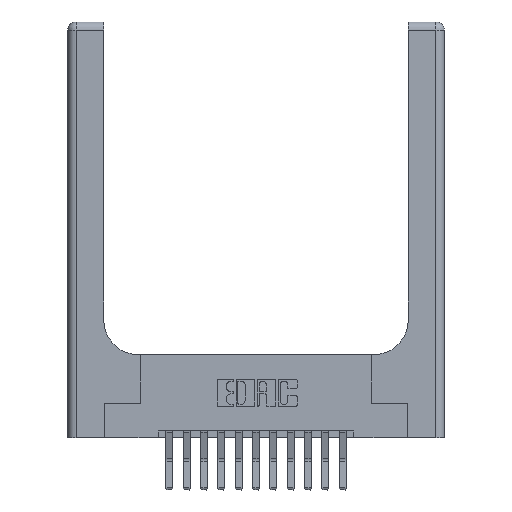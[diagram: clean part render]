
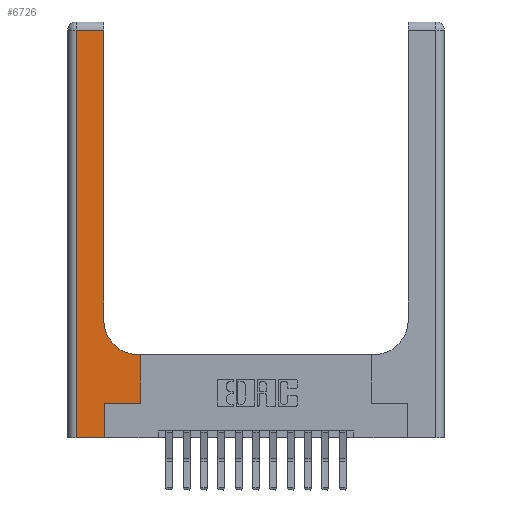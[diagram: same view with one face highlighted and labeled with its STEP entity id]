
A CAD part, top view. The second image highlights one B-rep face of the part: STEP entity #6726.
In plain terms, the highlighted planar face has unit normal (0, 0, 1).
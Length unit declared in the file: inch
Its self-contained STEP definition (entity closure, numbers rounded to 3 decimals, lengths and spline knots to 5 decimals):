
#40 = VECTOR ( 'NONE', #6164, 39.37008 ) ;
#179 = VECTOR ( 'NONE', #2635, 39.37008 ) ;
#310 = LINE ( 'NONE', #14817, #179 ) ;
#576 = ORIENTED_EDGE ( 'NONE', *, *, #7065, .T. ) ;
#774 = VECTOR ( 'NONE', #9963, 39.37008 ) ;
#799 = ORIENTED_EDGE ( 'NONE', *, *, #4863, .T. ) ;
#861 = VECTOR ( 'NONE', #8467, 39.37008 ) ;
#1094 = DIRECTION ( 'NONE',  ( 1., 0., 0. ) ) ;
#1190 = DIRECTION ( 'NONE',  ( 1., 0., 0. ) ) ;
#1558 = EDGE_CURVE ( 'NONE', #4758, #15224, #4155, .T. ) ;
#1905 = DIRECTION ( 'NONE',  ( 0., 0., -1. ) ) ;
#1984 = CARTESIAN_POINT ( 'NONE',  ( 0.265, 0., 0.37 ) ) ;
#2122 = ORIENTED_EDGE ( 'NONE', *, *, #2611, .T. ) ;
#2321 = LINE ( 'NONE', #9156, #13183 ) ;
#2480 = VERTEX_POINT ( 'NONE', #4492 ) ;
#2515 = EDGE_CURVE ( 'NONE', #2480, #12943, #10779, .T. ) ;
#2611 = EDGE_CURVE ( 'NONE', #15224, #6782, #4359, .T. ) ;
#2635 = DIRECTION ( 'NONE',  ( 0., 1., 0. ) ) ;
#2997 = LINE ( 'NONE', #5791, #774 ) ;
#3455 = CARTESIAN_POINT ( 'NONE',  ( 0.51, 0.85, 0.37 ) ) ;
#3461 = CARTESIAN_POINT ( 'NONE',  ( 0., 3., 0.37 ) ) ;
#3521 = CARTESIAN_POINT ( 'NONE',  ( 0.265, 0.25, 0.37 ) ) ;
#3657 = CARTESIAN_POINT ( 'NONE',  ( 0.528, 0.25, 0.37 ) ) ;
#4143 = EDGE_CURVE ( 'NONE', #16834, #12425, #2321, .T. ) ;
#4155 = LINE ( 'NONE', #9263, #8194 ) ;
#4359 = LINE ( 'NONE', #9868, #4423 ) ;
#4423 = VECTOR ( 'NONE', #8439, 39.37008 ) ;
#4476 = CARTESIAN_POINT ( 'NONE',  ( 0.265, 0., 0.37 ) ) ;
#4492 = CARTESIAN_POINT ( 'NONE',  ( 0.51, 0.6, 0.37 ) ) ;
#4731 = CARTESIAN_POINT ( 'NONE',  ( 0.06, 2.94, 0.37 ) ) ;
#4758 = VERTEX_POINT ( 'NONE', #4731 ) ;
#4863 = EDGE_CURVE ( 'NONE', #12943, #10801, #310, .T. ) ;
#5688 = CARTESIAN_POINT ( 'NONE',  ( 0.26, 0.85, 0.37 ) ) ;
#5791 = CARTESIAN_POINT ( 'NONE',  ( 0.26, 0.6, 0.37 ) ) ;
#6164 = DIRECTION ( 'NONE',  ( -1., 0., 0. ) ) ;
#6383 = EDGE_CURVE ( 'NONE', #10801, #4758, #15051, .T. ) ;
#6726 = ADVANCED_FACE ( 'NONE', ( #7409 ), #13890, .F. ) ;
#6782 = VERTEX_POINT ( 'NONE', #1984 ) ;
#7065 = EDGE_CURVE ( 'NONE', #6782, #16834, #15273, .T. ) ;
#7409 = FACE_OUTER_BOUND ( 'NONE', #8846, .T. ) ;
#7570 = EDGE_CURVE ( 'NONE', #12425, #8839, #15466, .T. ) ;
#7981 = ORIENTED_EDGE ( 'NONE', *, *, #10159, .T. ) ;
#8194 = VECTOR ( 'NONE', #11832, 39.37008 ) ;
#8236 = ORIENTED_EDGE ( 'NONE', *, *, #2515, .T. ) ;
#8439 = DIRECTION ( 'NONE',  ( 1., 0., 0. ) ) ;
#8467 = DIRECTION ( 'NONE',  ( 0., 1., 0. ) ) ;
#8839 = VERTEX_POINT ( 'NONE', #14017 ) ;
#8846 = EDGE_LOOP ( 'NONE', ( #799, #11122, #15072, #2122, #576, #13754, #10611, #7981, #8236 ) ) ;
#8929 = DIRECTION ( 'NONE',  ( 0., 1., 0. ) ) ;
#9156 = CARTESIAN_POINT ( 'NONE',  ( 0.265, 0.25, 0.37 ) ) ;
#9263 = CARTESIAN_POINT ( 'NONE',  ( 0.06, 3., 0.37 ) ) ;
#9868 = CARTESIAN_POINT ( 'NONE',  ( 0., 0., 0.37 ) ) ;
#9963 = DIRECTION ( 'NONE',  ( -1., 0., 0. ) ) ;
#10159 = EDGE_CURVE ( 'NONE', #8839, #2480, #2997, .T. ) ;
#10533 = CARTESIAN_POINT ( 'NONE',  ( 0.26, 2.94, 0.37 ) ) ;
#10611 = ORIENTED_EDGE ( 'NONE', *, *, #7570, .T. ) ;
#10779 = CIRCLE ( 'NONE', #15454, 0.25 ) ;
#10801 = VERTEX_POINT ( 'NONE', #10533 ) ;
#11122 = ORIENTED_EDGE ( 'NONE', *, *, #6383, .T. ) ;
#11248 = CARTESIAN_POINT ( 'NONE',  ( 0., 2.94, 0.37 ) ) ;
#11832 = DIRECTION ( 'NONE',  ( 0., -1., 0. ) ) ;
#12425 = VERTEX_POINT ( 'NONE', #15222 ) ;
#12532 = DIRECTION ( 'NONE',  ( -1., 0., 0. ) ) ;
#12943 = VERTEX_POINT ( 'NONE', #5688 ) ;
#13183 = VECTOR ( 'NONE', #1190, 39.37008 ) ;
#13754 = ORIENTED_EDGE ( 'NONE', *, *, #4143, .T. ) ;
#13890 = PLANE ( 'NONE',  #16319 ) ;
#13973 = DIRECTION ( 'NONE',  ( 0., 0., -1. ) ) ;
#14017 = CARTESIAN_POINT ( 'NONE',  ( 0.528, 0.6, 0.37 ) ) ;
#14045 = CARTESIAN_POINT ( 'NONE',  ( 0.06, 0., 0.37 ) ) ;
#14817 = CARTESIAN_POINT ( 'NONE',  ( 0.26, 3., 0.37 ) ) ;
#15051 = LINE ( 'NONE', #11248, #40 ) ;
#15072 = ORIENTED_EDGE ( 'NONE', *, *, #1558, .T. ) ;
#15222 = CARTESIAN_POINT ( 'NONE',  ( 0.528, 0.25, 0.37 ) ) ;
#15224 = VERTEX_POINT ( 'NONE', #14045 ) ;
#15273 = LINE ( 'NONE', #4476, #861 ) ;
#15454 = AXIS2_PLACEMENT_3D ( 'NONE', #3455, #13973, #1094 ) ;
#15466 = LINE ( 'NONE', #3657, #15823 ) ;
#15823 = VECTOR ( 'NONE', #8929, 39.37008 ) ;
#16319 = AXIS2_PLACEMENT_3D ( 'NONE', #3461, #1905, #12532 ) ;
#16834 = VERTEX_POINT ( 'NONE', #3521 ) ;
